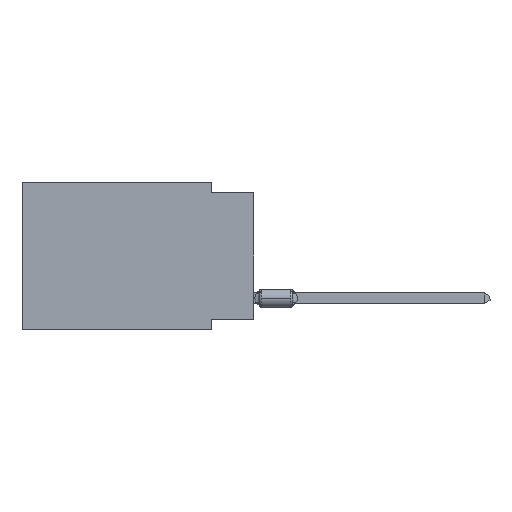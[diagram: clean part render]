
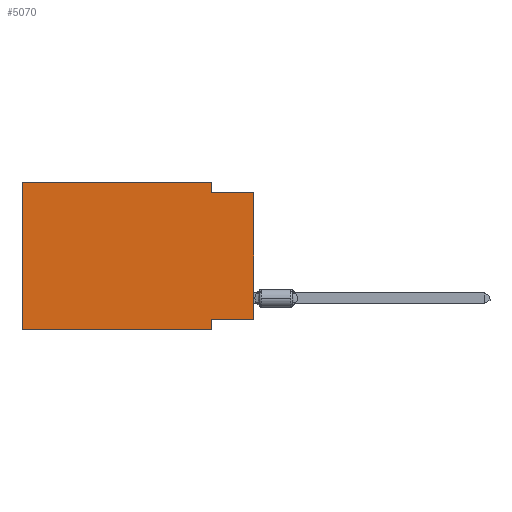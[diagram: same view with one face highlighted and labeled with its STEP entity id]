
A CAD part, left-side view. The second image highlights one B-rep face of the part: STEP entity #5070.
In plain terms, the highlighted planar face has unit normal (-1, 0, 0).
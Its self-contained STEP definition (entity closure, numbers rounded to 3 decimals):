
#1076 = CARTESIAN_POINT ( 'NONE',  ( 0., 13.97, -8.89 ) ) ;
#2784 = CARTESIAN_POINT ( 'NONE',  ( 0., 2.54, 0. ) ) ;
#3042 = EDGE_CURVE ( 'NONE', #21112, #14790, #15731, .T. ) ;
#3141 = ORIENTED_EDGE ( 'NONE', *, *, #7396, .F. ) ;
#3142 = EDGE_CURVE ( 'NONE', #20268, #8502, #12390, .T. ) ;
#3239 = CARTESIAN_POINT ( 'NONE',  ( 0., 0., -0.635 ) ) ;
#3349 = VECTOR ( 'NONE', #21126, 1000. ) ;
#3444 = CARTESIAN_POINT ( 'NONE',  ( 0., 0., -0.635 ) ) ;
#4841 = LINE ( 'NONE', #6663, #6001 ) ;
#5070 = ADVANCED_FACE ( 'NONE', ( #16309 ), #7900, .F. ) ;
#5495 = VECTOR ( 'NONE', #12814, 1000. ) ;
#5698 = CARTESIAN_POINT ( 'NONE',  ( 0., 0., 0. ) ) ;
#5751 = CARTESIAN_POINT ( 'NONE',  ( 0., 13.97, -8.89 ) ) ;
#5824 = VECTOR ( 'NONE', #17244, 1000. ) ;
#6001 = VECTOR ( 'NONE', #13652, 1000. ) ;
#6505 = ORIENTED_EDGE ( 'NONE', *, *, #16518, .F. ) ;
#6663 = CARTESIAN_POINT ( 'NONE',  ( 0., 0., -8.255 ) ) ;
#7286 = ORIENTED_EDGE ( 'NONE', *, *, #3042, .F. ) ;
#7396 = EDGE_CURVE ( 'NONE', #14790, #20268, #13537, .T. ) ;
#7563 = CARTESIAN_POINT ( 'NONE',  ( 0., 13.97, 0. ) ) ;
#7886 = ORIENTED_EDGE ( 'NONE', *, *, #3142, .F. ) ;
#7900 = PLANE ( 'NONE',  #14483 ) ;
#8347 = ORIENTED_EDGE ( 'NONE', *, *, #13209, .T. ) ;
#8377 = DIRECTION ( 'NONE',  ( 0., -1., 0. ) ) ;
#8502 = VERTEX_POINT ( 'NONE', #3239 ) ;
#8581 = VERTEX_POINT ( 'NONE', #18527 ) ;
#8774 = VECTOR ( 'NONE', #21091, 1000. ) ;
#9256 = LINE ( 'NONE', #5698, #5495 ) ;
#10964 = CARTESIAN_POINT ( 'NONE',  ( 0., 2.54, -8.89 ) ) ;
#12390 = LINE ( 'NONE', #3444, #3349 ) ;
#12414 = LINE ( 'NONE', #5751, #18928 ) ;
#12558 = VERTEX_POINT ( 'NONE', #1076 ) ;
#12673 = VERTEX_POINT ( 'NONE', #14078 ) ;
#12683 = EDGE_CURVE ( 'NONE', #12797, #12673, #17881, .T. ) ;
#12797 = VERTEX_POINT ( 'NONE', #19864 ) ;
#12814 = DIRECTION ( 'NONE',  ( 0., 0., 1. ) ) ;
#13209 = EDGE_CURVE ( 'NONE', #8581, #8502, #9256, .T. ) ;
#13537 = LINE ( 'NONE', #13872, #18931 ) ;
#13652 = DIRECTION ( 'NONE',  ( 0., 1., 0. ) ) ;
#13872 = CARTESIAN_POINT ( 'NONE',  ( 0., 2.54, 0. ) ) ;
#13928 = ORIENTED_EDGE ( 'NONE', *, *, #22112, .F. ) ;
#14078 = CARTESIAN_POINT ( 'NONE',  ( 0., 2.54, -8.89 ) ) ;
#14483 = AXIS2_PLACEMENT_3D ( 'NONE', #7563, #14566, #21559 ) ;
#14566 = DIRECTION ( 'NONE',  ( 1., 0., 0. ) ) ;
#14790 = VERTEX_POINT ( 'NONE', #2784 ) ;
#15075 = LINE ( 'NONE', #20663, #5824 ) ;
#15731 = LINE ( 'NONE', #20987, #18402 ) ;
#16309 = FACE_OUTER_BOUND ( 'NONE', #22249, .T. ) ;
#16315 = CARTESIAN_POINT ( 'NONE',  ( 0., 13.97, 0. ) ) ;
#16518 = EDGE_CURVE ( 'NONE', #8581, #12797, #4841, .T. ) ;
#16607 = ORIENTED_EDGE ( 'NONE', *, *, #12683, .F. ) ;
#17244 = DIRECTION ( 'NONE',  ( 0., 0., 1. ) ) ;
#17824 = DIRECTION ( 'NONE',  ( 0., -1., 0. ) ) ;
#17881 = LINE ( 'NONE', #10964, #8774 ) ;
#18402 = VECTOR ( 'NONE', #8377, 1000. ) ;
#18527 = CARTESIAN_POINT ( 'NONE',  ( 0., 0., -8.255 ) ) ;
#18742 = ORIENTED_EDGE ( 'NONE', *, *, #20017, .T. ) ;
#18928 = VECTOR ( 'NONE', #17824, 1000. ) ;
#18931 = VECTOR ( 'NONE', #20892, 1000. ) ;
#19864 = CARTESIAN_POINT ( 'NONE',  ( 0., 2.54, -8.255 ) ) ;
#20017 = EDGE_CURVE ( 'NONE', #12558, #12673, #12414, .T. ) ;
#20268 = VERTEX_POINT ( 'NONE', #20777 ) ;
#20663 = CARTESIAN_POINT ( 'NONE',  ( 0., 13.97, 0. ) ) ;
#20777 = CARTESIAN_POINT ( 'NONE',  ( 0., 2.54, -0.635 ) ) ;
#20892 = DIRECTION ( 'NONE',  ( 0., 0., -1. ) ) ;
#20987 = CARTESIAN_POINT ( 'NONE',  ( 0., 13.97, 0. ) ) ;
#21091 = DIRECTION ( 'NONE',  ( 0., 0., -1. ) ) ;
#21112 = VERTEX_POINT ( 'NONE', #16315 ) ;
#21126 = DIRECTION ( 'NONE',  ( 0., -1., 0. ) ) ;
#21559 = DIRECTION ( 'NONE',  ( 0., 0., -1. ) ) ;
#22112 = EDGE_CURVE ( 'NONE', #12558, #21112, #15075, .T. ) ;
#22249 = EDGE_LOOP ( 'NONE', ( #8347, #7886, #3141, #7286, #13928, #18742, #16607, #6505 ) ) ;
